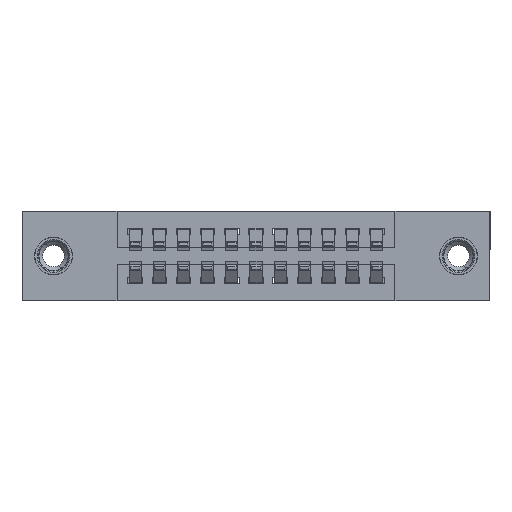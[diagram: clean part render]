
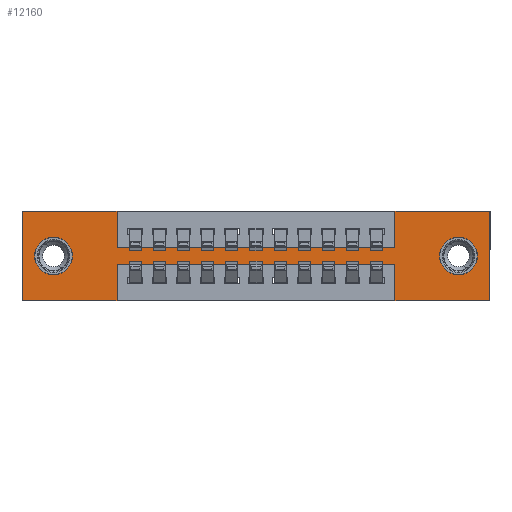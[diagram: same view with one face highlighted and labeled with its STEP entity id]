
A CAD part, front view. The second image highlights one B-rep face of the part: STEP entity #12160.
In plain terms, the highlighted planar face has unit normal (0, -1, 0).
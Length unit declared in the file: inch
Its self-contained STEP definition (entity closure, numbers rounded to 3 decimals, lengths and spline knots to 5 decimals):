
#9 = VECTOR ( 'NONE', #5387, 39.37008 ) ;
#11 = CARTESIAN_POINT ( 'NONE',  ( 0.3925, 0., -0.22 ) ) ;
#50 = CARTESIAN_POINT ( 'NONE',  ( 0.3925, 0., -0.15 ) ) ;
#182 = ORIENTED_EDGE ( 'NONE', *, *, #282, .T. ) ;
#237 = CARTESIAN_POINT ( 'NONE',  ( 1.935, 0., 0. ) ) ;
#244 = CARTESIAN_POINT ( 'NONE',  ( 1.5425, 0., -0.22 ) ) ;
#282 = EDGE_CURVE ( 'NONE', #500, #3644, #3276, .T. ) ;
#454 = VECTOR ( 'NONE', #4817, 39.37008 ) ;
#500 = VERTEX_POINT ( 'NONE', #13679 ) ;
#663 = DIRECTION ( 'NONE',  ( 0., 0., 1. ) ) ;
#699 = EDGE_CURVE ( 'NONE', #11913, #9414, #11396, .T. ) ;
#840 = LINE ( 'NONE', #7162, #11449 ) ;
#885 = EDGE_LOOP ( 'NONE', ( #14494, #7527, #11470, #10625, #5681, #8961, #3605, #10456, #1892, #17543, #10707, #15432 ) ) ;
#955 = CARTESIAN_POINT ( 'NONE',  ( 0.3925, 0., 0. ) ) ;
#1248 = CIRCLE ( 'NONE', #11798, 0.078 ) ;
#1482 = DIRECTION ( 'NONE',  ( -1., 0., 0. ) ) ;
#1570 = FACE_OUTER_BOUND ( 'NONE', #885, .T. ) ;
#1614 = CIRCLE ( 'NONE', #13541, 0.078 ) ;
#1824 = VERTEX_POINT ( 'NONE', #13207 ) ;
#1892 = ORIENTED_EDGE ( 'NONE', *, *, #16958, .F. ) ;
#1943 = VERTEX_POINT ( 'NONE', #4199 ) ;
#1953 = EDGE_CURVE ( 'NONE', #9207, #1943, #15071, .T. ) ;
#2088 = VECTOR ( 'NONE', #13011, 39.37008 ) ;
#2112 = ORIENTED_EDGE ( 'NONE', *, *, #8303, .T. ) ;
#2129 = EDGE_CURVE ( 'NONE', #17160, #4181, #13440, .T. ) ;
#2259 = CARTESIAN_POINT ( 'NONE',  ( 1.805, 0., -0.185 ) ) ;
#2798 = CARTESIAN_POINT ( 'NONE',  ( 0., 0., -0.37 ) ) ;
#2996 = VECTOR ( 'NONE', #8126, 39.37008 ) ;
#3058 = LINE ( 'NONE', #16984, #16547 ) ;
#3243 = EDGE_CURVE ( 'NONE', #9414, #11913, #1614, .T. ) ;
#3276 = CIRCLE ( 'NONE', #4514, 0.078 ) ;
#3297 = VERTEX_POINT ( 'NONE', #3862 ) ;
#3605 = ORIENTED_EDGE ( 'NONE', *, *, #15721, .F. ) ;
#3644 = VERTEX_POINT ( 'NONE', #3986 ) ;
#3691 = DIRECTION ( 'NONE',  ( 0., 0., -1. ) ) ;
#3727 = CARTESIAN_POINT ( 'NONE',  ( 0., 0., -0.37 ) ) ;
#3862 = CARTESIAN_POINT ( 'NONE',  ( 1.5425, 0., -0.37 ) ) ;
#3986 = CARTESIAN_POINT ( 'NONE',  ( 1.805, 0., -0.107 ) ) ;
#4132 = CARTESIAN_POINT ( 'NONE',  ( 0.13, 0., -0.263 ) ) ;
#4181 = VERTEX_POINT ( 'NONE', #955 ) ;
#4199 = CARTESIAN_POINT ( 'NONE',  ( 1.935, 0., -0.37 ) ) ;
#4228 = DIRECTION ( 'NONE',  ( 0., 0., 1. ) ) ;
#4460 = CARTESIAN_POINT ( 'NONE',  ( 0.13, 0., -0.185 ) ) ;
#4514 = AXIS2_PLACEMENT_3D ( 'NONE', #7466, #16815, #8818 ) ;
#4682 = CARTESIAN_POINT ( 'NONE',  ( 0., 0., -0.37 ) ) ;
#4695 = CARTESIAN_POINT ( 'NONE',  ( 0.13, 0., -0.107 ) ) ;
#4727 = DIRECTION ( 'NONE',  ( 0., 1., 0. ) ) ;
#4817 = DIRECTION ( 'NONE',  ( 0., 0., -1. ) ) ;
#4867 = LINE ( 'NONE', #3727, #15161 ) ;
#5354 = FACE_BOUND ( 'NONE', #14924, .T. ) ;
#5387 = DIRECTION ( 'NONE',  ( 1., 0., 0. ) ) ;
#5412 = EDGE_CURVE ( 'NONE', #14334, #12031, #840, .T. ) ;
#5672 = EDGE_CURVE ( 'NONE', #1824, #10683, #4867, .T. ) ;
#5678 = CARTESIAN_POINT ( 'NONE',  ( 0.3925, 0., -0.37 ) ) ;
#5681 = ORIENTED_EDGE ( 'NONE', *, *, #1953, .F. ) ;
#5683 = CARTESIAN_POINT ( 'NONE',  ( 1.5425, 0., -0.37 ) ) ;
#5958 = EDGE_CURVE ( 'NONE', #3297, #9364, #11428, .T. ) ;
#6127 = VECTOR ( 'NONE', #1482, 39.37008 ) ;
#6131 = PLANE ( 'NONE',  #6704 ) ;
#6424 = ORIENTED_EDGE ( 'NONE', *, *, #3243, .T. ) ;
#6441 = VERTEX_POINT ( 'NONE', #13683 ) ;
#6704 = AXIS2_PLACEMENT_3D ( 'NONE', #4682, #7470, #16820 ) ;
#6890 = CARTESIAN_POINT ( 'NONE',  ( 0., 0., 0. ) ) ;
#7020 = DIRECTION ( 'NONE',  ( 0., 0., -1. ) ) ;
#7028 = DIRECTION ( 'NONE',  ( 0., 0., 1. ) ) ;
#7162 = CARTESIAN_POINT ( 'NONE',  ( 0.3925, 0., -0.15 ) ) ;
#7466 = CARTESIAN_POINT ( 'NONE',  ( 1.805, 0., -0.185 ) ) ;
#7470 = DIRECTION ( 'NONE',  ( 0., -1., 0. ) ) ;
#7527 = ORIENTED_EDGE ( 'NONE', *, *, #13623, .F. ) ;
#7573 = CARTESIAN_POINT ( 'NONE',  ( 1.5425, 0., 0. ) ) ;
#8126 = DIRECTION ( 'NONE',  ( 1., 0., 0. ) ) ;
#8242 = VECTOR ( 'NONE', #7028, 39.37008 ) ;
#8249 = EDGE_CURVE ( 'NONE', #10683, #17160, #3058, .T. ) ;
#8303 = EDGE_CURVE ( 'NONE', #3644, #500, #1248, .T. ) ;
#8730 = AXIS2_PLACEMENT_3D ( 'NONE', #8820, #15061, #13656 ) ;
#8818 = DIRECTION ( 'NONE',  ( 0., 0., -1. ) ) ;
#8820 = CARTESIAN_POINT ( 'NONE',  ( 0.13, 0., -0.185 ) ) ;
#8916 = FACE_BOUND ( 'NONE', #16053, .T. ) ;
#8940 = VERTEX_POINT ( 'NONE', #10419 ) ;
#8961 = ORIENTED_EDGE ( 'NONE', *, *, #16530, .F. ) ;
#9207 = VERTEX_POINT ( 'NONE', #13635 ) ;
#9364 = VERTEX_POINT ( 'NONE', #244 ) ;
#9414 = VERTEX_POINT ( 'NONE', #4695 ) ;
#9895 = LINE ( 'NONE', #5678, #16134 ) ;
#10279 = LINE ( 'NONE', #7573, #2088 ) ;
#10388 = DIRECTION ( 'NONE',  ( 0., 0., -1. ) ) ;
#10419 = CARTESIAN_POINT ( 'NONE',  ( 0.3925, 0., -0.22 ) ) ;
#10456 = ORIENTED_EDGE ( 'NONE', *, *, #5412, .F. ) ;
#10625 = ORIENTED_EDGE ( 'NONE', *, *, #17641, .F. ) ;
#10683 = VERTEX_POINT ( 'NONE', #14123 ) ;
#10689 = LINE ( 'NONE', #12104, #9 ) ;
#10707 = ORIENTED_EDGE ( 'NONE', *, *, #8249, .F. ) ;
#10800 = ORIENTED_EDGE ( 'NONE', *, *, #699, .T. ) ;
#11084 = DIRECTION ( 'NONE',  ( -1., 0., 0. ) ) ;
#11287 = VECTOR ( 'NONE', #11084, 39.37008 ) ;
#11396 = CIRCLE ( 'NONE', #8730, 0.078 ) ;
#11428 = LINE ( 'NONE', #5683, #8242 ) ;
#11449 = VECTOR ( 'NONE', #16488, 39.37008 ) ;
#11470 = ORIENTED_EDGE ( 'NONE', *, *, #5958, .F. ) ;
#11557 = VECTOR ( 'NONE', #10388, 39.37008 ) ;
#11798 = AXIS2_PLACEMENT_3D ( 'NONE', #2259, #11853, #3691 ) ;
#11853 = DIRECTION ( 'NONE',  ( 0., 1., 0. ) ) ;
#11913 = VERTEX_POINT ( 'NONE', #4132 ) ;
#12031 = VERTEX_POINT ( 'NONE', #15157 ) ;
#12104 = CARTESIAN_POINT ( 'NONE',  ( 0., 0., 0. ) ) ;
#12160 = ADVANCED_FACE ( 'NONE', ( #8916, #5354, #1570 ), #6131, .T. ) ;
#12906 = CARTESIAN_POINT ( 'NONE',  ( 0.3925, 0., 0. ) ) ;
#13011 = DIRECTION ( 'NONE',  ( 0., 0., 1. ) ) ;
#13207 = CARTESIAN_POINT ( 'NONE',  ( 0.3925, 0., -0.37 ) ) ;
#13242 = DIRECTION ( 'NONE',  ( -1., 0., 0. ) ) ;
#13303 = LINE ( 'NONE', #11, #6127 ) ;
#13440 = LINE ( 'NONE', #6890, #2996 ) ;
#13541 = AXIS2_PLACEMENT_3D ( 'NONE', #4460, #4727, #4228 ) ;
#13623 = EDGE_CURVE ( 'NONE', #9364, #8940, #13303, .T. ) ;
#13635 = CARTESIAN_POINT ( 'NONE',  ( 1.935, 0., 0. ) ) ;
#13656 = DIRECTION ( 'NONE',  ( 0., 0., 1. ) ) ;
#13679 = CARTESIAN_POINT ( 'NONE',  ( 1.805, 0., -0.263 ) ) ;
#13683 = CARTESIAN_POINT ( 'NONE',  ( 1.5425, 0., 0. ) ) ;
#14123 = CARTESIAN_POINT ( 'NONE',  ( 0., 0., -0.37 ) ) ;
#14289 = EDGE_CURVE ( 'NONE', #8940, #1824, #9895, .T. ) ;
#14334 = VERTEX_POINT ( 'NONE', #50 ) ;
#14494 = ORIENTED_EDGE ( 'NONE', *, *, #14289, .F. ) ;
#14620 = LINE ( 'NONE', #12906, #454 ) ;
#14800 = LINE ( 'NONE', #2798, #11287 ) ;
#14924 = EDGE_LOOP ( 'NONE', ( #6424, #10800 ) ) ;
#15061 = DIRECTION ( 'NONE',  ( 0., 1., 0. ) ) ;
#15071 = LINE ( 'NONE', #237, #11557 ) ;
#15157 = CARTESIAN_POINT ( 'NONE',  ( 1.5425, 0., -0.15 ) ) ;
#15161 = VECTOR ( 'NONE', #13242, 39.37008 ) ;
#15432 = ORIENTED_EDGE ( 'NONE', *, *, #5672, .F. ) ;
#15721 = EDGE_CURVE ( 'NONE', #12031, #6441, #10279, .T. ) ;
#15951 = CARTESIAN_POINT ( 'NONE',  ( 0., 0., 0. ) ) ;
#16053 = EDGE_LOOP ( 'NONE', ( #2112, #182 ) ) ;
#16134 = VECTOR ( 'NONE', #7020, 39.37008 ) ;
#16488 = DIRECTION ( 'NONE',  ( 1., 0., 0. ) ) ;
#16530 = EDGE_CURVE ( 'NONE', #6441, #9207, #10689, .T. ) ;
#16547 = VECTOR ( 'NONE', #663, 39.37008 ) ;
#16815 = DIRECTION ( 'NONE',  ( 0., 1., 0. ) ) ;
#16820 = DIRECTION ( 'NONE',  ( 0., 0., -1. ) ) ;
#16958 = EDGE_CURVE ( 'NONE', #4181, #14334, #14620, .T. ) ;
#16984 = CARTESIAN_POINT ( 'NONE',  ( 0., 0., 0. ) ) ;
#17160 = VERTEX_POINT ( 'NONE', #15951 ) ;
#17543 = ORIENTED_EDGE ( 'NONE', *, *, #2129, .F. ) ;
#17641 = EDGE_CURVE ( 'NONE', #1943, #3297, #14800, .T. ) ;
